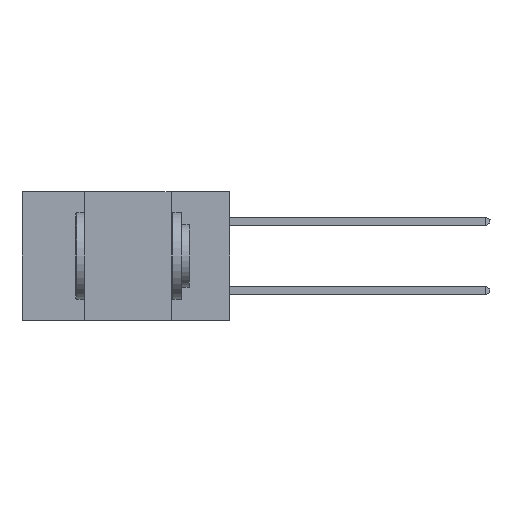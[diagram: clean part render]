
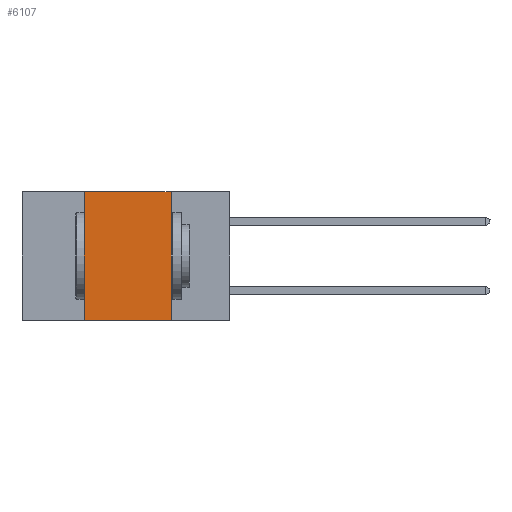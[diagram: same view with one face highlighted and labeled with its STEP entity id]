
A CAD part, left-side view. The second image highlights one B-rep face of the part: STEP entity #6107.
In plain terms, the highlighted planar face has unit normal (-1, 0, 0).
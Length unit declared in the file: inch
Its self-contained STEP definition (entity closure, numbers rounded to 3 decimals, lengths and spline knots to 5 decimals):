
#379 = VECTOR ( 'NONE', #2947, 39.37008 ) ;
#1736 = ORIENTED_EDGE ( 'NONE', *, *, #4578, .F. ) ;
#1770 = ORIENTED_EDGE ( 'NONE', *, *, #19819, .F. ) ;
#1976 = ORIENTED_EDGE ( 'NONE', *, *, #11087, .F. ) ;
#2251 = FACE_OUTER_BOUND ( 'NONE', #7983, .T. ) ;
#2947 = DIRECTION ( 'NONE',  ( 0., -1., 0. ) ) ;
#3103 = CARTESIAN_POINT ( 'NONE',  ( 0., 0.6, -0.37 ) ) ;
#4199 = LINE ( 'NONE', #17987, #9340 ) ;
#4578 = EDGE_CURVE ( 'NONE', #19621, #9462, #4199, .T. ) ;
#4986 = LINE ( 'NONE', #3103, #379 ) ;
#5488 = EDGE_CURVE ( 'NONE', #16829, #6599, #4986, .T. ) ;
#5553 = CARTESIAN_POINT ( 'NONE',  ( 0., 0.17, -0.37 ) ) ;
#6107 = ADVANCED_FACE ( 'NONE', ( #2251 ), #9362, .F. ) ;
#6599 = VERTEX_POINT ( 'NONE', #5553 ) ;
#7087 = DIRECTION ( 'NONE',  ( 0., 0., -1. ) ) ;
#7545 = DIRECTION ( 'NONE',  ( 1., 0., 0. ) ) ;
#7885 = LINE ( 'NONE', #14299, #12259 ) ;
#7983 = EDGE_LOOP ( 'NONE', ( #1976, #1736, #1770, #18641 ) ) ;
#8326 = CARTESIAN_POINT ( 'NONE',  ( 0., 0.42, 0. ) ) ;
#8726 = CARTESIAN_POINT ( 'NONE',  ( 0., 0.42, -0.37 ) ) ;
#9340 = VECTOR ( 'NONE', #12848, 39.37008 ) ;
#9362 = PLANE ( 'NONE',  #9397 ) ;
#9394 = LINE ( 'NONE', #17149, #17257 ) ;
#9397 = AXIS2_PLACEMENT_3D ( 'NONE', #21469, #7545, #7087 ) ;
#9462 = VERTEX_POINT ( 'NONE', #20994 ) ;
#11087 = EDGE_CURVE ( 'NONE', #9462, #6599, #9394, .T. ) ;
#12259 = VECTOR ( 'NONE', #17853, 39.37008 ) ;
#12848 = DIRECTION ( 'NONE',  ( 0., -1., 0. ) ) ;
#14299 = CARTESIAN_POINT ( 'NONE',  ( 0., 0.42, 0. ) ) ;
#16829 = VERTEX_POINT ( 'NONE', #8726 ) ;
#17149 = CARTESIAN_POINT ( 'NONE',  ( 0., 0.17, 0. ) ) ;
#17257 = VECTOR ( 'NONE', #20707, 39.37008 ) ;
#17853 = DIRECTION ( 'NONE',  ( 0., 0., 1. ) ) ;
#17987 = CARTESIAN_POINT ( 'NONE',  ( 0., 0.6, 0. ) ) ;
#18641 = ORIENTED_EDGE ( 'NONE', *, *, #5488, .T. ) ;
#19621 = VERTEX_POINT ( 'NONE', #8326 ) ;
#19819 = EDGE_CURVE ( 'NONE', #16829, #19621, #7885, .T. ) ;
#20707 = DIRECTION ( 'NONE',  ( 0., 0., -1. ) ) ;
#20994 = CARTESIAN_POINT ( 'NONE',  ( 0., 0.17, 0. ) ) ;
#21469 = CARTESIAN_POINT ( 'NONE',  ( 0., 0.6, 0. ) ) ;
